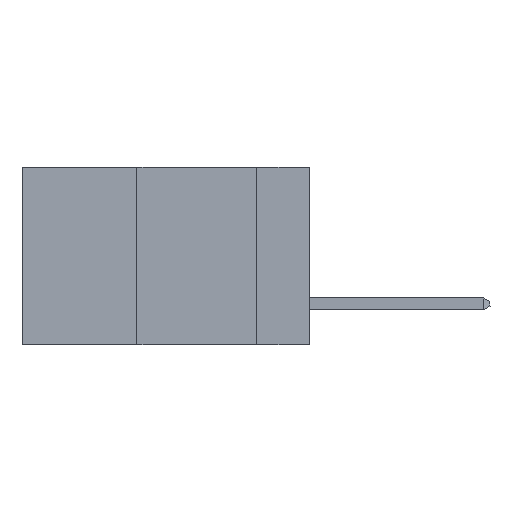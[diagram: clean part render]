
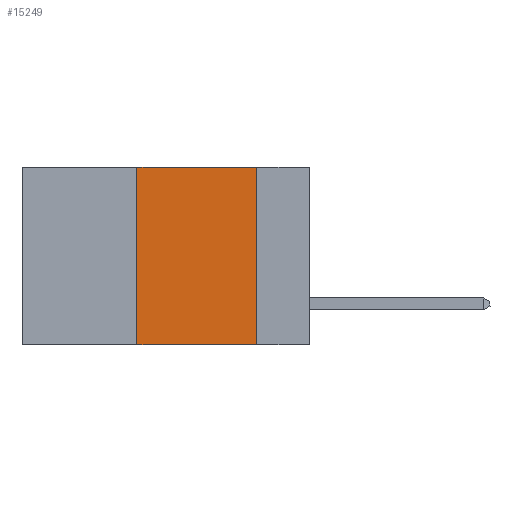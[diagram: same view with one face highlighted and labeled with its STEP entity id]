
A CAD part, left-side view. The second image highlights one B-rep face of the part: STEP entity #15249.
In plain terms, the highlighted planar face has unit normal (-1, 0, 0).
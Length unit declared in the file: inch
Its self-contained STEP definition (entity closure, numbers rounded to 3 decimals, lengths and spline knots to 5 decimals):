
#204 = VERTEX_POINT ( 'NONE', #2971 ) ;
#684 = FACE_OUTER_BOUND ( 'NONE', #9190, .T. ) ;
#734 = VECTOR ( 'NONE', #17210, 39.37008 ) ;
#2571 = ORIENTED_EDGE ( 'NONE', *, *, #9803, .F. ) ;
#2731 = AXIS2_PLACEMENT_3D ( 'NONE', #3907, #5550, #16608 ) ;
#2971 = CARTESIAN_POINT ( 'NONE',  ( 0., 0.36, -0.37 ) ) ;
#3190 = ORIENTED_EDGE ( 'NONE', *, *, #17063, .F. ) ;
#3458 = VERTEX_POINT ( 'NONE', #3719 ) ;
#3719 = CARTESIAN_POINT ( 'NONE',  ( 0., 0.36, 0. ) ) ;
#3907 = CARTESIAN_POINT ( 'NONE',  ( 0., 0.6, 0. ) ) ;
#4941 = EDGE_CURVE ( 'NONE', #204, #9242, #5103, .T. ) ;
#5103 = LINE ( 'NONE', #17146, #734 ) ;
#5311 = CARTESIAN_POINT ( 'NONE',  ( 0., 0.11, 0. ) ) ;
#5385 = EDGE_CURVE ( 'NONE', #3458, #16445, #9754, .T. ) ;
#5550 = DIRECTION ( 'NONE',  ( 1., 0., 0. ) ) ;
#5629 = CARTESIAN_POINT ( 'NONE',  ( 0., 0.6, 0. ) ) ;
#5931 = DIRECTION ( 'NONE',  ( 0., 0., 1. ) ) ;
#7211 = DIRECTION ( 'NONE',  ( 0., -1., 0. ) ) ;
#8687 = VECTOR ( 'NONE', #5931, 39.37008 ) ;
#8761 = VECTOR ( 'NONE', #7211, 39.37008 ) ;
#9190 = EDGE_LOOP ( 'NONE', ( #3190, #9367, #2571, #17159 ) ) ;
#9242 = VERTEX_POINT ( 'NONE', #18690 ) ;
#9367 = ORIENTED_EDGE ( 'NONE', *, *, #5385, .F. ) ;
#9754 = LINE ( 'NONE', #5629, #8761 ) ;
#9803 = EDGE_CURVE ( 'NONE', #204, #3458, #17148, .T. ) ;
#10666 = LINE ( 'NONE', #19426, #18624 ) ;
#11512 = DIRECTION ( 'NONE',  ( 0., 0., -1. ) ) ;
#13415 = PLANE ( 'NONE',  #2731 ) ;
#13803 = CARTESIAN_POINT ( 'NONE',  ( 0., 0.36, 0. ) ) ;
#15249 = ADVANCED_FACE ( 'NONE', ( #684 ), #13415, .F. ) ;
#16445 = VERTEX_POINT ( 'NONE', #5311 ) ;
#16608 = DIRECTION ( 'NONE',  ( 0., 0., -1. ) ) ;
#17063 = EDGE_CURVE ( 'NONE', #16445, #9242, #10666, .T. ) ;
#17146 = CARTESIAN_POINT ( 'NONE',  ( 0., 0.6, -0.37 ) ) ;
#17148 = LINE ( 'NONE', #13803, #8687 ) ;
#17159 = ORIENTED_EDGE ( 'NONE', *, *, #4941, .T. ) ;
#17210 = DIRECTION ( 'NONE',  ( 0., -1., 0. ) ) ;
#18624 = VECTOR ( 'NONE', #11512, 39.37008 ) ;
#18690 = CARTESIAN_POINT ( 'NONE',  ( 0., 0.11, -0.37 ) ) ;
#19426 = CARTESIAN_POINT ( 'NONE',  ( 0., 0.11, 0. ) ) ;
